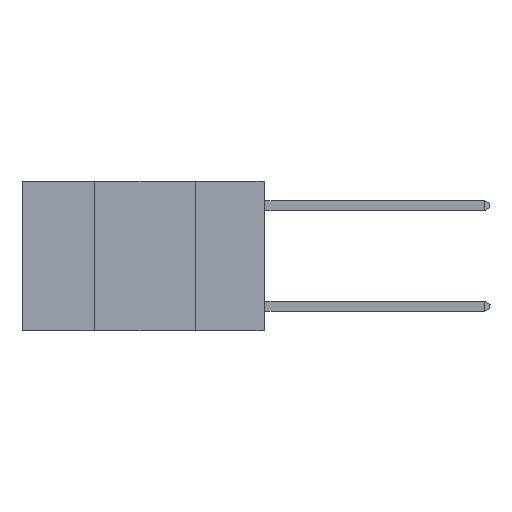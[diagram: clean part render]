
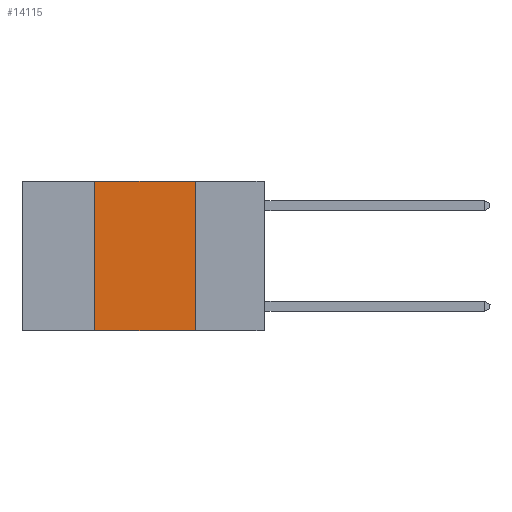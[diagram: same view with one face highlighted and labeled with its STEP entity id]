
A CAD part, left-side view. The second image highlights one B-rep face of the part: STEP entity #14115.
In plain terms, the highlighted planar face has unit normal (-1, 0, 0).
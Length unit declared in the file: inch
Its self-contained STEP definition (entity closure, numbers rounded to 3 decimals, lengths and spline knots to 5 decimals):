
#1751 = ORIENTED_EDGE ( 'NONE', *, *, #2052, .F. ) ;
#2052 = EDGE_CURVE ( 'NONE', #15862, #6971, #13708, .T. ) ;
#2124 = VECTOR ( 'NONE', #4865, 39.37008 ) ;
#2836 = CARTESIAN_POINT ( 'NONE',  ( 0., 0.6, 0. ) ) ;
#3623 = FACE_OUTER_BOUND ( 'NONE', #6360, .T. ) ;
#4519 = DIRECTION ( 'NONE',  ( 0., 0., -1. ) ) ;
#4721 = CARTESIAN_POINT ( 'NONE',  ( 0., 0.42, 0. ) ) ;
#4865 = DIRECTION ( 'NONE',  ( 0., -1., 0. ) ) ;
#5107 = PLANE ( 'NONE',  #13350 ) ;
#5389 = CARTESIAN_POINT ( 'NONE',  ( 0., 0.42, 0. ) ) ;
#5740 = LINE ( 'NONE', #5917, #6002 ) ;
#5917 = CARTESIAN_POINT ( 'NONE',  ( 0., 0.17, 0. ) ) ;
#6002 = VECTOR ( 'NONE', #4519, 39.37008 ) ;
#6165 = CARTESIAN_POINT ( 'NONE',  ( 0., 0.6, -0.37 ) ) ;
#6235 = DIRECTION ( 'NONE',  ( 0., 0., -1. ) ) ;
#6326 = LINE ( 'NONE', #6165, #2124 ) ;
#6360 = EDGE_LOOP ( 'NONE', ( #14272, #9239, #1751, #16969 ) ) ;
#6971 = VERTEX_POINT ( 'NONE', #4721 ) ;
#7420 = EDGE_CURVE ( 'NONE', #15214, #9058, #5740, .T. ) ;
#7996 = DIRECTION ( 'NONE',  ( 0., 0., 1. ) ) ;
#8147 = DIRECTION ( 'NONE',  ( 0., -1., 0. ) ) ;
#8936 = DIRECTION ( 'NONE',  ( 1., 0., 0. ) ) ;
#9058 = VERTEX_POINT ( 'NONE', #9067 ) ;
#9067 = CARTESIAN_POINT ( 'NONE',  ( 0., 0.17, -0.37 ) ) ;
#9239 = ORIENTED_EDGE ( 'NONE', *, *, #10362, .F. ) ;
#9727 = VECTOR ( 'NONE', #7996, 39.37008 ) ;
#9960 = EDGE_CURVE ( 'NONE', #15862, #9058, #6326, .T. ) ;
#10317 = CARTESIAN_POINT ( 'NONE',  ( 0., 0.6, 0. ) ) ;
#10362 = EDGE_CURVE ( 'NONE', #6971, #15214, #14759, .T. ) ;
#11028 = VECTOR ( 'NONE', #8147, 39.37008 ) ;
#12214 = CARTESIAN_POINT ( 'NONE',  ( 0., 0.17, 0. ) ) ;
#13350 = AXIS2_PLACEMENT_3D ( 'NONE', #10317, #8936, #6235 ) ;
#13708 = LINE ( 'NONE', #5389, #9727 ) ;
#14115 = ADVANCED_FACE ( 'NONE', ( #3623 ), #5107, .F. ) ;
#14272 = ORIENTED_EDGE ( 'NONE', *, *, #7420, .F. ) ;
#14759 = LINE ( 'NONE', #2836, #11028 ) ;
#15214 = VERTEX_POINT ( 'NONE', #12214 ) ;
#15862 = VERTEX_POINT ( 'NONE', #16363 ) ;
#16363 = CARTESIAN_POINT ( 'NONE',  ( 0., 0.42, -0.37 ) ) ;
#16969 = ORIENTED_EDGE ( 'NONE', *, *, #9960, .T. ) ;
